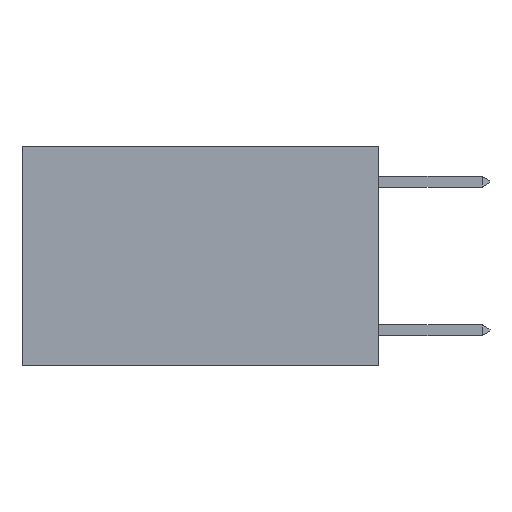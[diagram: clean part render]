
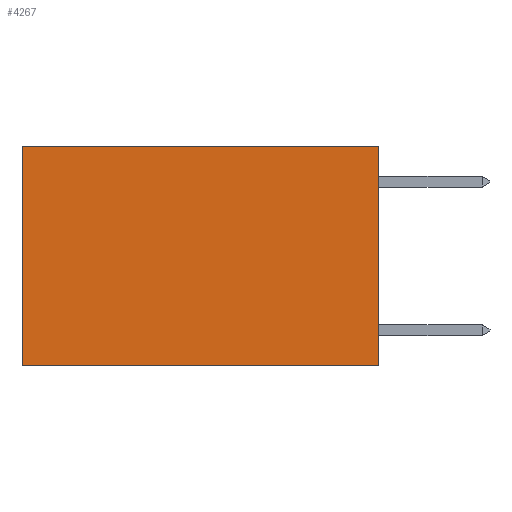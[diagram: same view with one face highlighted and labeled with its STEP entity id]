
A CAD part, left-side view. The second image highlights one B-rep face of the part: STEP entity #4267.
In plain terms, the highlighted planar face has unit normal (-1, 0, 0).
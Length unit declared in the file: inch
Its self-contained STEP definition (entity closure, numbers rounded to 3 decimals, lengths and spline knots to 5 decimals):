
#48 = CARTESIAN_POINT ( 'NONE',  ( 0.2625, 0., -0.37 ) ) ;
#461 = ORIENTED_EDGE ( 'NONE', *, *, #6478, .T. ) ;
#1137 = ORIENTED_EDGE ( 'NONE', *, *, #5834, .F. ) ;
#1561 = DIRECTION ( 'NONE',  ( 0., 1., 0. ) ) ;
#1921 = EDGE_LOOP ( 'NONE', ( #461, #5601, #1137, #3010 ) ) ;
#2120 = EDGE_CURVE ( 'NONE', #2569, #4856, #4362, .T. ) ;
#2182 = CARTESIAN_POINT ( 'NONE',  ( 0.2625, 0.6, -0.37 ) ) ;
#2493 = CARTESIAN_POINT ( 'NONE',  ( 0.2625, 0.6, 0. ) ) ;
#2569 = VERTEX_POINT ( 'NONE', #48 ) ;
#2654 = LINE ( 'NONE', #6481, #5761 ) ;
#2729 = VERTEX_POINT ( 'NONE', #5267 ) ;
#3010 = ORIENTED_EDGE ( 'NONE', *, *, #4137, .T. ) ;
#3388 = VECTOR ( 'NONE', #1561, 39.37008 ) ;
#3704 = DIRECTION ( 'NONE',  ( 0., 1., 0. ) ) ;
#3973 = CARTESIAN_POINT ( 'NONE',  ( 0.2625, 0., 0. ) ) ;
#4137 = EDGE_CURVE ( 'NONE', #7353, #2729, #2654, .T. ) ;
#4267 = ADVANCED_FACE ( 'NONE', ( #5042 ), #5931, .F. ) ;
#4362 = LINE ( 'NONE', #6983, #3388 ) ;
#4398 = VECTOR ( 'NONE', #7846, 39.37008 ) ;
#4512 = VECTOR ( 'NONE', #5537, 39.37008 ) ;
#4856 = VERTEX_POINT ( 'NONE', #2182 ) ;
#5042 = FACE_OUTER_BOUND ( 'NONE', #1921, .T. ) ;
#5267 = CARTESIAN_POINT ( 'NONE',  ( 0.2625, 0.6, 0. ) ) ;
#5522 = CARTESIAN_POINT ( 'NONE',  ( 0.2625, 0., 0. ) ) ;
#5537 = DIRECTION ( 'NONE',  ( 0., 0., -1. ) ) ;
#5601 = ORIENTED_EDGE ( 'NONE', *, *, #2120, .F. ) ;
#5761 = VECTOR ( 'NONE', #3704, 39.37008 ) ;
#5834 = EDGE_CURVE ( 'NONE', #7353, #2569, #7872, .T. ) ;
#5931 = PLANE ( 'NONE',  #6631 ) ;
#5993 = DIRECTION ( 'NONE',  ( 0., 0., -1. ) ) ;
#6021 = DIRECTION ( 'NONE',  ( 1., 0., 0. ) ) ;
#6478 = EDGE_CURVE ( 'NONE', #2729, #4856, #7038, .T. ) ;
#6481 = CARTESIAN_POINT ( 'NONE',  ( 0.2625, 0., 0. ) ) ;
#6631 = AXIS2_PLACEMENT_3D ( 'NONE', #3973, #6021, #5993 ) ;
#6983 = CARTESIAN_POINT ( 'NONE',  ( 0.2625, 0., -0.37 ) ) ;
#7001 = CARTESIAN_POINT ( 'NONE',  ( 0.2625, 0., 0. ) ) ;
#7038 = LINE ( 'NONE', #2493, #4398 ) ;
#7353 = VERTEX_POINT ( 'NONE', #5522 ) ;
#7846 = DIRECTION ( 'NONE',  ( 0., 0., -1. ) ) ;
#7872 = LINE ( 'NONE', #7001, #4512 ) ;
